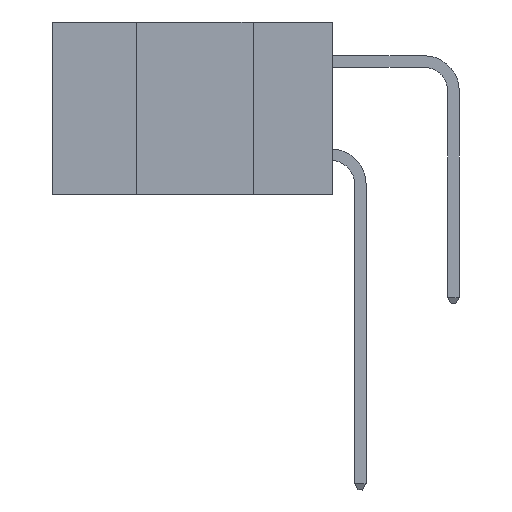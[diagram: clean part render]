
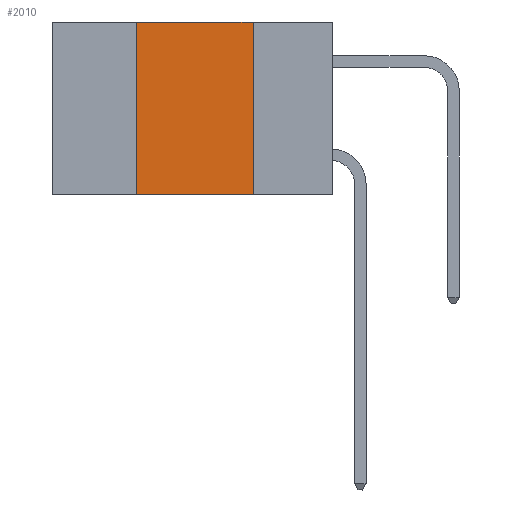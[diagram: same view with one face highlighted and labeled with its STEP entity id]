
A CAD part, left-side view. The second image highlights one B-rep face of the part: STEP entity #2010.
In plain terms, the highlighted planar face has unit normal (-1, 0, 0).
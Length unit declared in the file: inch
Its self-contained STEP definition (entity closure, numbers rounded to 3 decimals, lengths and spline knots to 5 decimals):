
#610 = CARTESIAN_POINT ( 'NONE',  ( 0., 0.17, 0. ) ) ;
#747 = VECTOR ( 'NONE', #9685, 39.37008 ) ;
#965 = EDGE_CURVE ( 'NONE', #11274, #4734, #6875, .T. ) ;
#1546 = CARTESIAN_POINT ( 'NONE',  ( 0., 0.42, -0.37 ) ) ;
#1896 = DIRECTION ( 'NONE',  ( 1., 0., 0. ) ) ;
#2010 = ADVANCED_FACE ( 'NONE', ( #11807 ), #17096, .F. ) ;
#3113 = CARTESIAN_POINT ( 'NONE',  ( 0., 0.6, 0. ) ) ;
#3203 = ORIENTED_EDGE ( 'NONE', *, *, #6430, .T. ) ;
#3267 = CARTESIAN_POINT ( 'NONE',  ( 0., 0.6, -0.37 ) ) ;
#3450 = AXIS2_PLACEMENT_3D ( 'NONE', #3113, #1896, #4236 ) ;
#4117 = DIRECTION ( 'NONE',  ( 0., -1., 0. ) ) ;
#4236 = DIRECTION ( 'NONE',  ( 0., 0., -1. ) ) ;
#4292 = LINE ( 'NONE', #4383, #747 ) ;
#4307 = VECTOR ( 'NONE', #13842, 39.37008 ) ;
#4383 = CARTESIAN_POINT ( 'NONE',  ( 0., 0.17, -0.37 ) ) ;
#4537 = ORIENTED_EDGE ( 'NONE', *, *, #7764, .F. ) ;
#4734 = VERTEX_POINT ( 'NONE', #610 ) ;
#5256 = VERTEX_POINT ( 'NONE', #14251 ) ;
#5471 = VECTOR ( 'NONE', #6874, 39.37008 ) ;
#5698 = VERTEX_POINT ( 'NONE', #1546 ) ;
#6430 = EDGE_CURVE ( 'NONE', #5698, #5256, #11077, .T. ) ;
#6874 = DIRECTION ( 'NONE',  ( 0., 0., 1. ) ) ;
#6875 = LINE ( 'NONE', #16168, #15423 ) ;
#7034 = CARTESIAN_POINT ( 'NONE',  ( 0., 0.42, -0.37 ) ) ;
#7407 = ORIENTED_EDGE ( 'NONE', *, *, #965, .F. ) ;
#7764 = EDGE_CURVE ( 'NONE', #4734, #5256, #4292, .T. ) ;
#8092 = EDGE_CURVE ( 'NONE', #5698, #11274, #12104, .T. ) ;
#9685 = DIRECTION ( 'NONE',  ( 0., 0., -1. ) ) ;
#11077 = LINE ( 'NONE', #3267, #4307 ) ;
#11274 = VERTEX_POINT ( 'NONE', #13137 ) ;
#11807 = FACE_OUTER_BOUND ( 'NONE', #13688, .T. ) ;
#12104 = LINE ( 'NONE', #7034, #5471 ) ;
#13137 = CARTESIAN_POINT ( 'NONE',  ( 0., 0.42, 0. ) ) ;
#13688 = EDGE_LOOP ( 'NONE', ( #4537, #7407, #15096, #3203 ) ) ;
#13842 = DIRECTION ( 'NONE',  ( 0., -1., 0. ) ) ;
#14251 = CARTESIAN_POINT ( 'NONE',  ( 0., 0.17, -0.37 ) ) ;
#15096 = ORIENTED_EDGE ( 'NONE', *, *, #8092, .F. ) ;
#15423 = VECTOR ( 'NONE', #4117, 39.37008 ) ;
#16168 = CARTESIAN_POINT ( 'NONE',  ( 0., 0.6, 0. ) ) ;
#17096 = PLANE ( 'NONE',  #3450 ) ;
